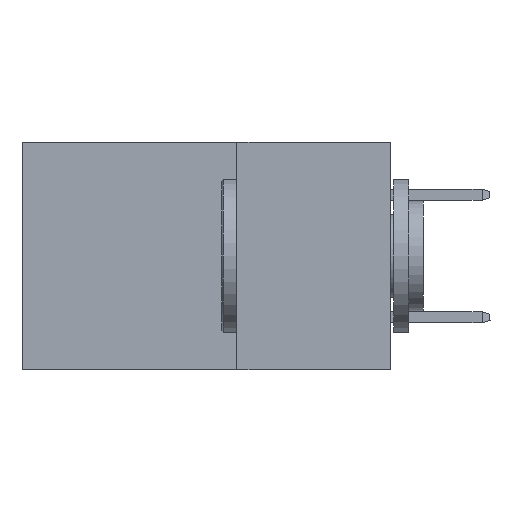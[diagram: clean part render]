
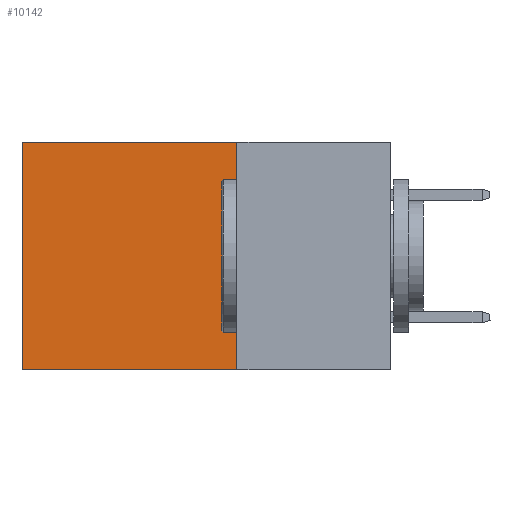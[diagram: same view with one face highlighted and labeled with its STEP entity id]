
A CAD part, left-side view. The second image highlights one B-rep face of the part: STEP entity #10142.
In plain terms, the highlighted planar face has unit normal (-1, 0, 0).
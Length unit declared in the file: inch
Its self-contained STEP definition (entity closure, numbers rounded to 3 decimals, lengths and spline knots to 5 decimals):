
#847 = VECTOR ( 'NONE', #5326, 39.37008 ) ;
#1134 = ORIENTED_EDGE ( 'NONE', *, *, #11056, .F. ) ;
#1854 = DIRECTION ( 'NONE',  ( 0., 1., 0. ) ) ;
#2133 = CARTESIAN_POINT ( 'NONE',  ( 0.2875, 0.25, -0.37 ) ) ;
#2868 = VECTOR ( 'NONE', #1854, 39.37008 ) ;
#3027 = DIRECTION ( 'NONE',  ( 0., 1., 0. ) ) ;
#3999 = CARTESIAN_POINT ( 'NONE',  ( 0.2875, 0.25, -0.37 ) ) ;
#4035 = PLANE ( 'NONE',  #9486 ) ;
#4372 = DIRECTION ( 'NONE',  ( 1., 0., 0. ) ) ;
#4746 = EDGE_LOOP ( 'NONE', ( #9680, #12487, #1134, #6523 ) ) ;
#4762 = DIRECTION ( 'NONE',  ( 0., 0., -1. ) ) ;
#5163 = VERTEX_POINT ( 'NONE', #2133 ) ;
#5326 = DIRECTION ( 'NONE',  ( 0., 0., -1. ) ) ;
#5465 = VERTEX_POINT ( 'NONE', #10782 ) ;
#5573 = EDGE_CURVE ( 'NONE', #5465, #9427, #10722, .T. ) ;
#6523 = ORIENTED_EDGE ( 'NONE', *, *, #15263, .T. ) ;
#6801 = VERTEX_POINT ( 'NONE', #14378 ) ;
#8065 = CARTESIAN_POINT ( 'NONE',  ( 0.2875, 0.25, 0. ) ) ;
#8269 = CARTESIAN_POINT ( 'NONE',  ( 0.2875, 0.6, 0. ) ) ;
#9193 = LINE ( 'NONE', #3999, #15692 ) ;
#9427 = VERTEX_POINT ( 'NONE', #16260 ) ;
#9428 = CARTESIAN_POINT ( 'NONE',  ( 0.2875, 0.25, 0. ) ) ;
#9486 = AXIS2_PLACEMENT_3D ( 'NONE', #8065, #4372, #4762 ) ;
#9680 = ORIENTED_EDGE ( 'NONE', *, *, #5573, .T. ) ;
#9708 = VECTOR ( 'NONE', #13487, 39.37008 ) ;
#10142 = ADVANCED_FACE ( 'NONE', ( #15437 ), #4035, .F. ) ;
#10547 = LINE ( 'NONE', #16786, #847 ) ;
#10722 = LINE ( 'NONE', #8269, #9708 ) ;
#10782 = CARTESIAN_POINT ( 'NONE',  ( 0.2875, 0.6, 0. ) ) ;
#11004 = LINE ( 'NONE', #9428, #2868 ) ;
#11056 = EDGE_CURVE ( 'NONE', #6801, #5163, #10547, .T. ) ;
#12487 = ORIENTED_EDGE ( 'NONE', *, *, #13665, .F. ) ;
#13487 = DIRECTION ( 'NONE',  ( 0., 0., -1. ) ) ;
#13665 = EDGE_CURVE ( 'NONE', #5163, #9427, #9193, .T. ) ;
#14378 = CARTESIAN_POINT ( 'NONE',  ( 0.2875, 0.25, 0. ) ) ;
#15263 = EDGE_CURVE ( 'NONE', #6801, #5465, #11004, .T. ) ;
#15437 = FACE_OUTER_BOUND ( 'NONE', #4746, .T. ) ;
#15692 = VECTOR ( 'NONE', #3027, 39.37008 ) ;
#16260 = CARTESIAN_POINT ( 'NONE',  ( 0.2875, 0.6, -0.37 ) ) ;
#16786 = CARTESIAN_POINT ( 'NONE',  ( 0.2875, 0.25, 0. ) ) ;
